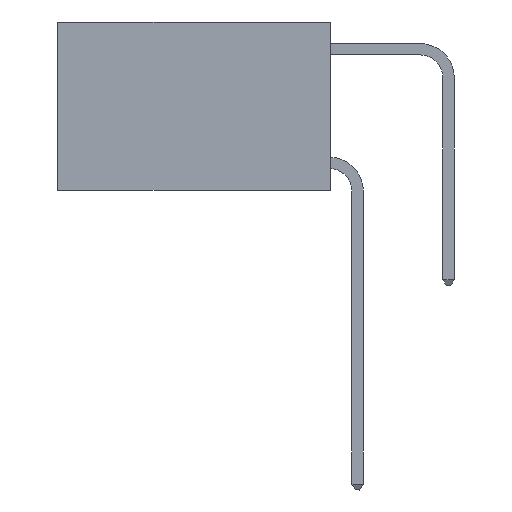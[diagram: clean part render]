
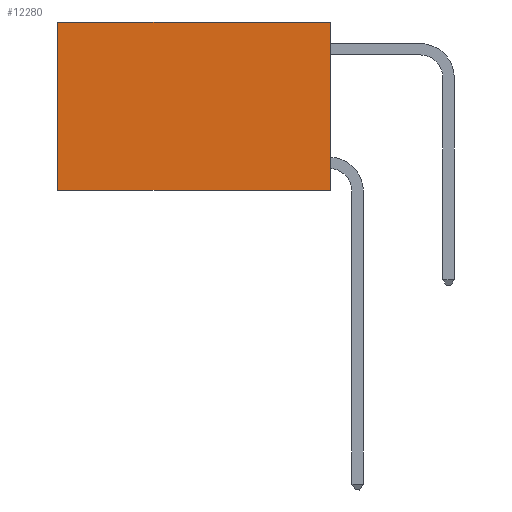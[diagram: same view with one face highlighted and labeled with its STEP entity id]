
A CAD part, left-side view. The second image highlights one B-rep face of the part: STEP entity #12280.
In plain terms, the highlighted planar face has unit normal (-1, 0, 0).
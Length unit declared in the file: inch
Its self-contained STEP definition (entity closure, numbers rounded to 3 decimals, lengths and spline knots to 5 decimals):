
#1251 = LINE ( 'NONE', #16850, #9150 ) ;
#1580 = EDGE_CURVE ( 'NONE', #19942, #10717, #19495, .T. ) ;
#2372 = EDGE_CURVE ( 'NONE', #16154, #12143, #1251, .T. ) ;
#2410 = ORIENTED_EDGE ( 'NONE', *, *, #1580, .T. ) ;
#2660 = CARTESIAN_POINT ( 'NONE',  ( 0.2625, 0.6, 0. ) ) ;
#3231 = CARTESIAN_POINT ( 'NONE',  ( 0.2625, 0.6, -0.37 ) ) ;
#3495 = CARTESIAN_POINT ( 'NONE',  ( 0.2625, 0., 0. ) ) ;
#4296 = DIRECTION ( 'NONE',  ( 0., 0., -1. ) ) ;
#4902 = EDGE_CURVE ( 'NONE', #19942, #16154, #6771, .T. ) ;
#6771 = LINE ( 'NONE', #12140, #10445 ) ;
#6915 = CARTESIAN_POINT ( 'NONE',  ( 0.2625, 0., 0. ) ) ;
#7493 = ORIENTED_EDGE ( 'NONE', *, *, #4902, .F. ) ;
#8257 = DIRECTION ( 'NONE',  ( 1., 0., 0. ) ) ;
#9006 = EDGE_LOOP ( 'NONE', ( #15721, #17297, #7493, #2410 ) ) ;
#9050 = DIRECTION ( 'NONE',  ( 0., 0., -1. ) ) ;
#9150 = VECTOR ( 'NONE', #16339, 39.37008 ) ;
#9528 = VECTOR ( 'NONE', #4296, 39.37008 ) ;
#10011 = LINE ( 'NONE', #2660, #9528 ) ;
#10445 = VECTOR ( 'NONE', #9050, 39.37008 ) ;
#10717 = VERTEX_POINT ( 'NONE', #16749 ) ;
#11098 = AXIS2_PLACEMENT_3D ( 'NONE', #3495, #8257, #19005 ) ;
#11229 = FACE_OUTER_BOUND ( 'NONE', #9006, .T. ) ;
#11508 = DIRECTION ( 'NONE',  ( 0., 1., 0. ) ) ;
#12140 = CARTESIAN_POINT ( 'NONE',  ( 0.2625, 0., 0. ) ) ;
#12143 = VERTEX_POINT ( 'NONE', #3231 ) ;
#12280 = ADVANCED_FACE ( 'NONE', ( #11229 ), #17427, .F. ) ;
#12624 = EDGE_CURVE ( 'NONE', #10717, #12143, #10011, .T. ) ;
#15721 = ORIENTED_EDGE ( 'NONE', *, *, #12624, .T. ) ;
#16154 = VERTEX_POINT ( 'NONE', #18525 ) ;
#16339 = DIRECTION ( 'NONE',  ( 0., 1., 0. ) ) ;
#16749 = CARTESIAN_POINT ( 'NONE',  ( 0.2625, 0.6, 0. ) ) ;
#16850 = CARTESIAN_POINT ( 'NONE',  ( 0.2625, 0., -0.37 ) ) ;
#17297 = ORIENTED_EDGE ( 'NONE', *, *, #2372, .F. ) ;
#17427 = PLANE ( 'NONE',  #11098 ) ;
#18525 = CARTESIAN_POINT ( 'NONE',  ( 0.2625, 0., -0.37 ) ) ;
#19005 = DIRECTION ( 'NONE',  ( 0., 0., -1. ) ) ;
#19263 = CARTESIAN_POINT ( 'NONE',  ( 0.2625, 0., 0. ) ) ;
#19495 = LINE ( 'NONE', #19263, #19965 ) ;
#19942 = VERTEX_POINT ( 'NONE', #6915 ) ;
#19965 = VECTOR ( 'NONE', #11508, 39.37008 ) ;
